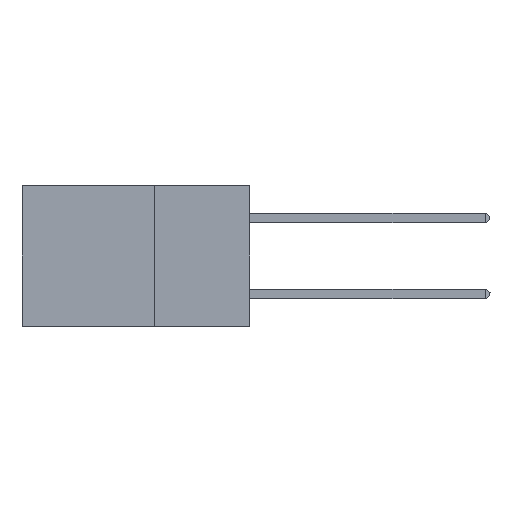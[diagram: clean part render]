
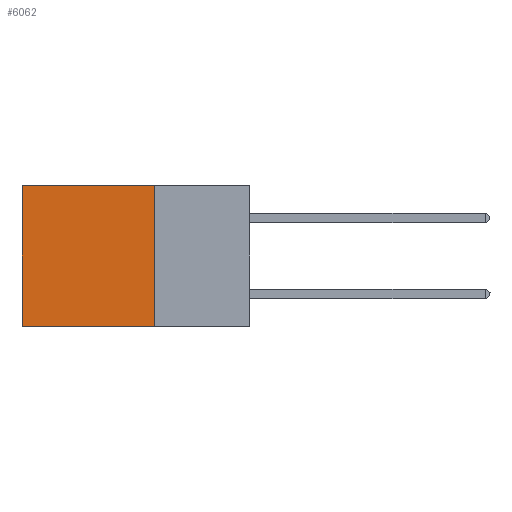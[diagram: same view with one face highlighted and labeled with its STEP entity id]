
A CAD part, left-side view. The second image highlights one B-rep face of the part: STEP entity #6062.
In plain terms, the highlighted planar face has unit normal (-1, 0, 0).
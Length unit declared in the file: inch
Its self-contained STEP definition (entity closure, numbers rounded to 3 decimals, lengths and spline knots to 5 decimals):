
#233 = VERTEX_POINT ( 'NONE', #11188 ) ;
#334 = EDGE_CURVE ( 'NONE', #22805, #3505, #9957, .T. ) ;
#880 = CARTESIAN_POINT ( 'NONE',  ( 0.2875, 0.25, 0. ) ) ;
#951 = EDGE_CURVE ( 'NONE', #21108, #233, #5329, .T. ) ;
#1345 = VECTOR ( 'NONE', #4858, 39.37008 ) ;
#1904 = DIRECTION ( 'NONE',  ( 1., 0., 0. ) ) ;
#3472 = AXIS2_PLACEMENT_3D ( 'NONE', #22114, #1904, #18349 ) ;
#3505 = VERTEX_POINT ( 'NONE', #20535 ) ;
#3598 = CARTESIAN_POINT ( 'NONE',  ( 0.2875, 0.25, -0.37 ) ) ;
#4632 = FACE_OUTER_BOUND ( 'NONE', #13920, .T. ) ;
#4858 = DIRECTION ( 'NONE',  ( 0., 0., -1. ) ) ;
#5329 = LINE ( 'NONE', #18222, #12847 ) ;
#6062 = ADVANCED_FACE ( 'NONE', ( #4632 ), #21888, .F. ) ;
#8076 = CARTESIAN_POINT ( 'NONE',  ( 0.2875, 0.25, 0. ) ) ;
#8585 = EDGE_CURVE ( 'NONE', #21108, #22805, #19086, .T. ) ;
#8671 = ORIENTED_EDGE ( 'NONE', *, *, #334, .F. ) ;
#9261 = ORIENTED_EDGE ( 'NONE', *, *, #19236, .T. ) ;
#9957 = LINE ( 'NONE', #22277, #23225 ) ;
#10523 = CARTESIAN_POINT ( 'NONE',  ( 0.2875, 0.6, 0. ) ) ;
#10720 = DIRECTION ( 'NONE',  ( 0., 1., 0. ) ) ;
#11114 = DIRECTION ( 'NONE',  ( 0., 1., 0. ) ) ;
#11188 = CARTESIAN_POINT ( 'NONE',  ( 0.2875, 0.6, 0. ) ) ;
#12847 = VECTOR ( 'NONE', #11114, 39.37008 ) ;
#13920 = EDGE_LOOP ( 'NONE', ( #9261, #8671, #18451, #15106 ) ) ;
#14188 = VECTOR ( 'NONE', #17424, 39.37008 ) ;
#15106 = ORIENTED_EDGE ( 'NONE', *, *, #951, .T. ) ;
#17424 = DIRECTION ( 'NONE',  ( 0., 0., -1. ) ) ;
#18222 = CARTESIAN_POINT ( 'NONE',  ( 0.2875, 0.25, 0. ) ) ;
#18349 = DIRECTION ( 'NONE',  ( 0., 0., -1. ) ) ;
#18451 = ORIENTED_EDGE ( 'NONE', *, *, #8585, .F. ) ;
#19086 = LINE ( 'NONE', #8076, #14188 ) ;
#19236 = EDGE_CURVE ( 'NONE', #233, #3505, #19800, .T. ) ;
#19800 = LINE ( 'NONE', #10523, #1345 ) ;
#20535 = CARTESIAN_POINT ( 'NONE',  ( 0.2875, 0.6, -0.37 ) ) ;
#21108 = VERTEX_POINT ( 'NONE', #880 ) ;
#21888 = PLANE ( 'NONE',  #3472 ) ;
#22114 = CARTESIAN_POINT ( 'NONE',  ( 0.2875, 0.25, 0. ) ) ;
#22277 = CARTESIAN_POINT ( 'NONE',  ( 0.2875, 0.25, -0.37 ) ) ;
#22805 = VERTEX_POINT ( 'NONE', #3598 ) ;
#23225 = VECTOR ( 'NONE', #10720, 39.37008 ) ;
